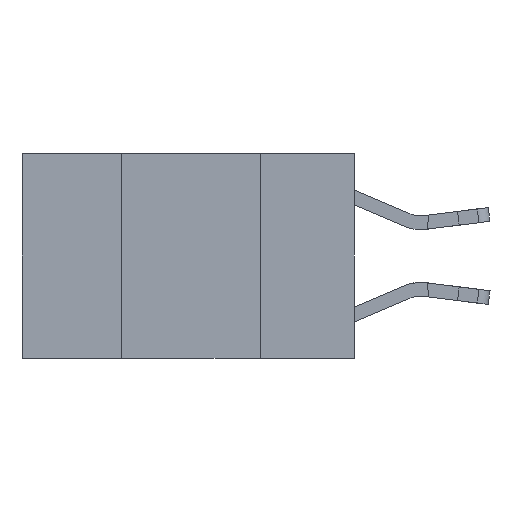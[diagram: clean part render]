
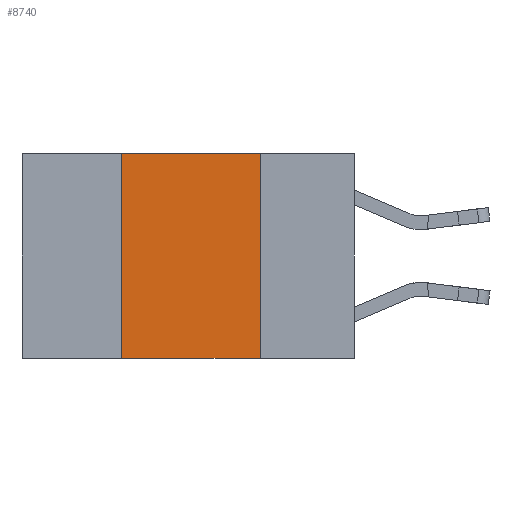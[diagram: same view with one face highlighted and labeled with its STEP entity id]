
A CAD part, left-side view. The second image highlights one B-rep face of the part: STEP entity #8740.
In plain terms, the highlighted planar face has unit normal (-1, 0, 0).
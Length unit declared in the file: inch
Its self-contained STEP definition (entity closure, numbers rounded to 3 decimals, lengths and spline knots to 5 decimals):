
#469 = EDGE_CURVE ( 'NONE', #20638, #2844, #12676, .T. ) ;
#1059 = ORIENTED_EDGE ( 'NONE', *, *, #9348, .T. ) ;
#1460 = CARTESIAN_POINT ( 'NONE',  ( 0., 0.6, 0. ) ) ;
#1994 = VECTOR ( 'NONE', #14704, 39.37008 ) ;
#2844 = VERTEX_POINT ( 'NONE', #12763 ) ;
#3351 = PLANE ( 'NONE',  #17745 ) ;
#4776 = VECTOR ( 'NONE', #24809, 39.37008 ) ;
#4990 = FACE_OUTER_BOUND ( 'NONE', #22271, .T. ) ;
#5425 = DIRECTION ( 'NONE',  ( 1., 0., 0. ) ) ;
#5715 = ORIENTED_EDGE ( 'NONE', *, *, #469, .F. ) ;
#7339 = CARTESIAN_POINT ( 'NONE',  ( 0., 0.17, 0. ) ) ;
#8740 = ADVANCED_FACE ( 'NONE', ( #4990 ), #3351, .F. ) ;
#9348 = EDGE_CURVE ( 'NONE', #22737, #13392, #12961, .T. ) ;
#9733 = CARTESIAN_POINT ( 'NONE',  ( 0., 0.42, -0.37 ) ) ;
#10032 = LINE ( 'NONE', #7339, #4776 ) ;
#10546 = CARTESIAN_POINT ( 'NONE',  ( 0., 0.17, -0.37 ) ) ;
#11873 = LINE ( 'NONE', #22448, #1994 ) ;
#12676 = LINE ( 'NONE', #21438, #24229 ) ;
#12763 = CARTESIAN_POINT ( 'NONE',  ( 0., 0.17, 0. ) ) ;
#12961 = LINE ( 'NONE', #20806, #22096 ) ;
#13392 = VERTEX_POINT ( 'NONE', #10546 ) ;
#14704 = DIRECTION ( 'NONE',  ( 0., 0., 1. ) ) ;
#15240 = EDGE_CURVE ( 'NONE', #2844, #13392, #10032, .T. ) ;
#15455 = CARTESIAN_POINT ( 'NONE',  ( 0., 0.42, 0. ) ) ;
#16125 = ORIENTED_EDGE ( 'NONE', *, *, #22403, .F. ) ;
#17745 = AXIS2_PLACEMENT_3D ( 'NONE', #1460, #5425, #19140 ) ;
#19140 = DIRECTION ( 'NONE',  ( 0., 0., -1. ) ) ;
#19480 = DIRECTION ( 'NONE',  ( 0., -1., 0. ) ) ;
#20638 = VERTEX_POINT ( 'NONE', #15455 ) ;
#20806 = CARTESIAN_POINT ( 'NONE',  ( 0., 0.6, -0.37 ) ) ;
#21438 = CARTESIAN_POINT ( 'NONE',  ( 0., 0.6, 0. ) ) ;
#22096 = VECTOR ( 'NONE', #23088, 39.37008 ) ;
#22271 = EDGE_LOOP ( 'NONE', ( #25193, #5715, #16125, #1059 ) ) ;
#22403 = EDGE_CURVE ( 'NONE', #22737, #20638, #11873, .T. ) ;
#22448 = CARTESIAN_POINT ( 'NONE',  ( 0., 0.42, 0. ) ) ;
#22737 = VERTEX_POINT ( 'NONE', #9733 ) ;
#23088 = DIRECTION ( 'NONE',  ( 0., -1., 0. ) ) ;
#24229 = VECTOR ( 'NONE', #19480, 39.37008 ) ;
#24809 = DIRECTION ( 'NONE',  ( 0., 0., -1. ) ) ;
#25193 = ORIENTED_EDGE ( 'NONE', *, *, #15240, .F. ) ;
